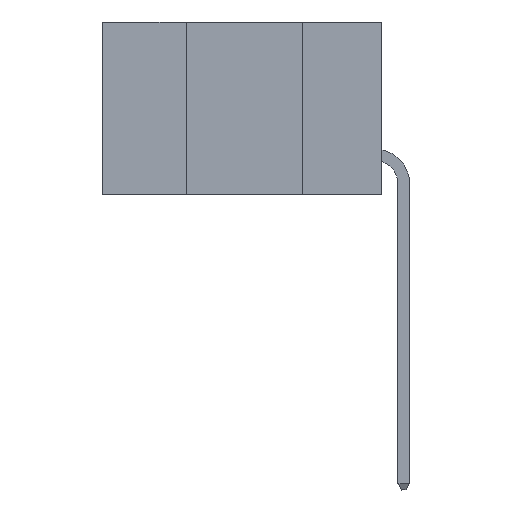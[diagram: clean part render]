
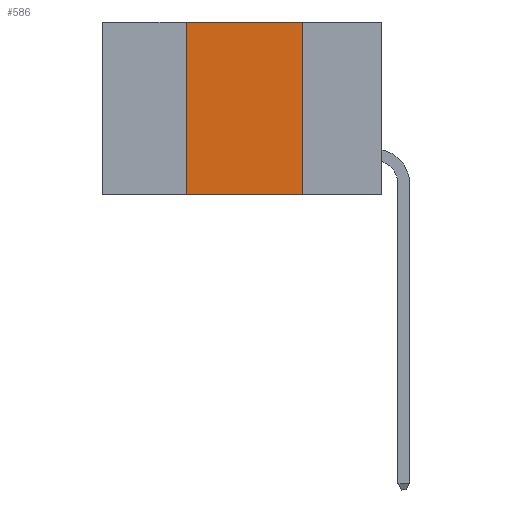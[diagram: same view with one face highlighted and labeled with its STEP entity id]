
A CAD part, left-side view. The second image highlights one B-rep face of the part: STEP entity #586.
In plain terms, the highlighted planar face has unit normal (-1, 0, 0).
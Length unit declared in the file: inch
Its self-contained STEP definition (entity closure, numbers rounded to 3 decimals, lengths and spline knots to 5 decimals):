
#208 = CARTESIAN_POINT ( 'NONE',  ( 0., 0.42, 0. ) ) ;
#254 = VERTEX_POINT ( 'NONE', #10657 ) ;
#449 = AXIS2_PLACEMENT_3D ( 'NONE', #14859, #4369, #18149 ) ;
#586 = ADVANCED_FACE ( 'NONE', ( #13601 ), #13606, .F. ) ;
#862 = VECTOR ( 'NONE', #14700, 39.37008 ) ;
#1390 = CARTESIAN_POINT ( 'NONE',  ( 0., 0.17, -0.37 ) ) ;
#2630 = CARTESIAN_POINT ( 'NONE',  ( 0., 0.42, 0. ) ) ;
#3481 = CARTESIAN_POINT ( 'NONE',  ( 0., 0.6, -0.37 ) ) ;
#4049 = DIRECTION ( 'NONE',  ( 0., 0., -1. ) ) ;
#4290 = EDGE_CURVE ( 'NONE', #15431, #17457, #17770, .T. ) ;
#4369 = DIRECTION ( 'NONE',  ( 1., 0., 0. ) ) ;
#6114 = EDGE_LOOP ( 'NONE', ( #12033, #6736, #16090, #19069 ) ) ;
#6736 = ORIENTED_EDGE ( 'NONE', *, *, #8691, .F. ) ;
#8691 = EDGE_CURVE ( 'NONE', #17457, #254, #16184, .T. ) ;
#8774 = VECTOR ( 'NONE', #4049, 39.37008 ) ;
#9070 = VECTOR ( 'NONE', #9635, 39.37008 ) ;
#9634 = VECTOR ( 'NONE', #16902, 39.37008 ) ;
#9635 = DIRECTION ( 'NONE',  ( 0., -1., 0. ) ) ;
#10639 = CARTESIAN_POINT ( 'NONE',  ( 0., 0.6, 0. ) ) ;
#10657 = CARTESIAN_POINT ( 'NONE',  ( 0., 0.17, 0. ) ) ;
#11449 = CARTESIAN_POINT ( 'NONE',  ( 0., 0.42, -0.37 ) ) ;
#12033 = ORIENTED_EDGE ( 'NONE', *, *, #18105, .F. ) ;
#13508 = LINE ( 'NONE', #3481, #9070 ) ;
#13601 = FACE_OUTER_BOUND ( 'NONE', #6114, .T. ) ;
#13606 = PLANE ( 'NONE',  #449 ) ;
#14397 = CARTESIAN_POINT ( 'NONE',  ( 0., 0.17, 0. ) ) ;
#14700 = DIRECTION ( 'NONE',  ( 0., 0., 1. ) ) ;
#14856 = VERTEX_POINT ( 'NONE', #1390 ) ;
#14859 = CARTESIAN_POINT ( 'NONE',  ( 0., 0.6, 0. ) ) ;
#15320 = EDGE_CURVE ( 'NONE', #15431, #14856, #13508, .T. ) ;
#15431 = VERTEX_POINT ( 'NONE', #11449 ) ;
#16090 = ORIENTED_EDGE ( 'NONE', *, *, #4290, .F. ) ;
#16184 = LINE ( 'NONE', #10639, #9634 ) ;
#16902 = DIRECTION ( 'NONE',  ( 0., -1., 0. ) ) ;
#17457 = VERTEX_POINT ( 'NONE', #208 ) ;
#17770 = LINE ( 'NONE', #2630, #862 ) ;
#18105 = EDGE_CURVE ( 'NONE', #254, #14856, #18169, .T. ) ;
#18149 = DIRECTION ( 'NONE',  ( 0., 0., -1. ) ) ;
#18169 = LINE ( 'NONE', #14397, #8774 ) ;
#19069 = ORIENTED_EDGE ( 'NONE', *, *, #15320, .T. ) ;
